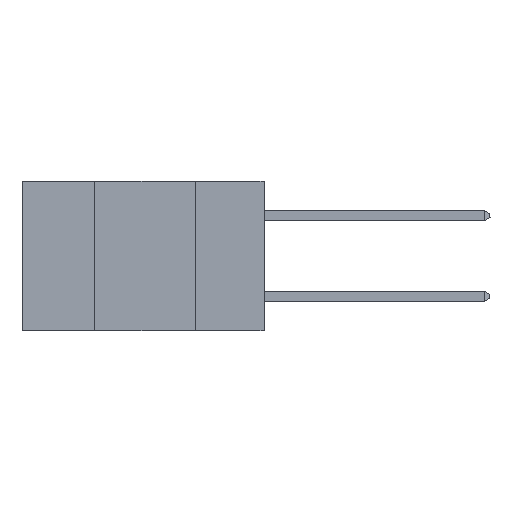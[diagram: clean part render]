
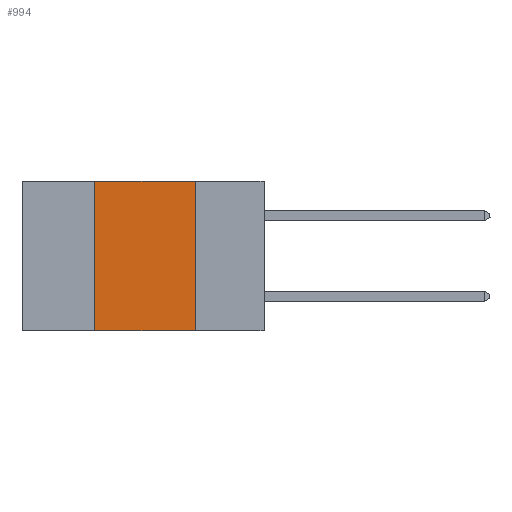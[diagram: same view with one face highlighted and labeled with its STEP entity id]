
A CAD part, left-side view. The second image highlights one B-rep face of the part: STEP entity #994.
In plain terms, the highlighted planar face has unit normal (-1, 0, 0).
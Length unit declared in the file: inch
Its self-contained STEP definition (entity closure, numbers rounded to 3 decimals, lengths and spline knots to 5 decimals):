
#368 = VECTOR ( 'NONE', #4004, 39.37008 ) ;
#450 = VECTOR ( 'NONE', #13828, 39.37008 ) ;
#759 = LINE ( 'NONE', #12761, #368 ) ;
#850 = DIRECTION ( 'NONE',  ( 0., 0., -1. ) ) ;
#994 = ADVANCED_FACE ( 'NONE', ( #2011 ), #13833, .F. ) ;
#999 = ORIENTED_EDGE ( 'NONE', *, *, #13382, .T. ) ;
#1082 = VERTEX_POINT ( 'NONE', #14962 ) ;
#1227 = VECTOR ( 'NONE', #13522, 39.37008 ) ;
#1373 = VERTEX_POINT ( 'NONE', #1702 ) ;
#1702 = CARTESIAN_POINT ( 'NONE',  ( 0., 0.17, -0.37 ) ) ;
#1894 = EDGE_LOOP ( 'NONE', ( #5266, #14961, #7301, #999 ) ) ;
#2011 = FACE_OUTER_BOUND ( 'NONE', #1894, .T. ) ;
#3514 = CARTESIAN_POINT ( 'NONE',  ( 0., 0.42, 0. ) ) ;
#4004 = DIRECTION ( 'NONE',  ( 0., -1., 0. ) ) ;
#4904 = CARTESIAN_POINT ( 'NONE',  ( 0., 0.6, 0. ) ) ;
#5266 = ORIENTED_EDGE ( 'NONE', *, *, #11770, .F. ) ;
#5492 = EDGE_CURVE ( 'NONE', #1082, #6384, #11910, .T. ) ;
#6079 = CARTESIAN_POINT ( 'NONE',  ( 0., 0.17, 0. ) ) ;
#6384 = VERTEX_POINT ( 'NONE', #7385 ) ;
#6410 = VERTEX_POINT ( 'NONE', #6079 ) ;
#7301 = ORIENTED_EDGE ( 'NONE', *, *, #5492, .F. ) ;
#7385 = CARTESIAN_POINT ( 'NONE',  ( 0., 0.42, 0. ) ) ;
#8177 = EDGE_CURVE ( 'NONE', #6384, #6410, #16288, .T. ) ;
#8485 = DIRECTION ( 'NONE',  ( 1., 0., 0. ) ) ;
#10897 = VECTOR ( 'NONE', #16380, 39.37008 ) ;
#11037 = CARTESIAN_POINT ( 'NONE',  ( 0., 0.17, 0. ) ) ;
#11125 = CARTESIAN_POINT ( 'NONE',  ( 0., 0.6, 0. ) ) ;
#11770 = EDGE_CURVE ( 'NONE', #6410, #1373, #13215, .T. ) ;
#11910 = LINE ( 'NONE', #3514, #10897 ) ;
#12259 = AXIS2_PLACEMENT_3D ( 'NONE', #11125, #8485, #850 ) ;
#12761 = CARTESIAN_POINT ( 'NONE',  ( 0., 0.6, -0.37 ) ) ;
#13215 = LINE ( 'NONE', #11037, #1227 ) ;
#13382 = EDGE_CURVE ( 'NONE', #1082, #1373, #759, .T. ) ;
#13522 = DIRECTION ( 'NONE',  ( 0., 0., -1. ) ) ;
#13828 = DIRECTION ( 'NONE',  ( 0., -1., 0. ) ) ;
#13833 = PLANE ( 'NONE',  #12259 ) ;
#14961 = ORIENTED_EDGE ( 'NONE', *, *, #8177, .F. ) ;
#14962 = CARTESIAN_POINT ( 'NONE',  ( 0., 0.42, -0.37 ) ) ;
#16288 = LINE ( 'NONE', #4904, #450 ) ;
#16380 = DIRECTION ( 'NONE',  ( 0., 0., 1. ) ) ;
